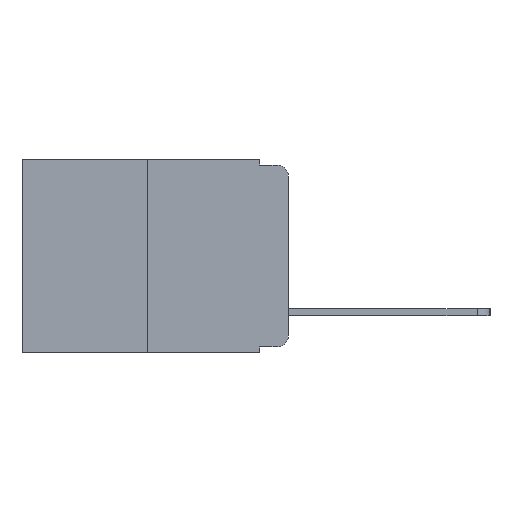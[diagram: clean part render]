
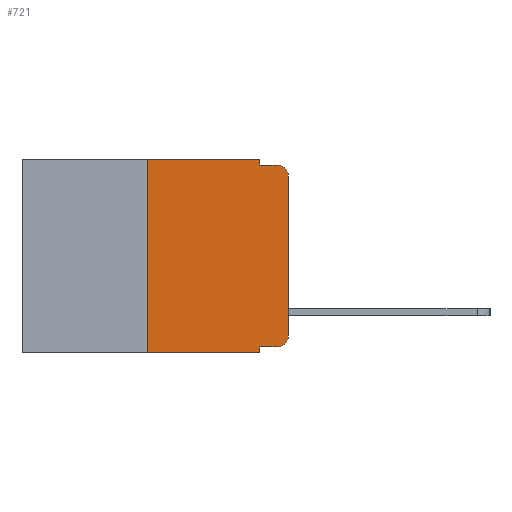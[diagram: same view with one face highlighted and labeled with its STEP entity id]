
A CAD part, left-side view. The second image highlights one B-rep face of the part: STEP entity #721.
In plain terms, the highlighted planar face has unit normal (-1, 0, 0).
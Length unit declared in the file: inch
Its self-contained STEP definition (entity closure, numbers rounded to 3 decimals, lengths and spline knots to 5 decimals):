
#57 = VECTOR ( 'NONE', #714, 39.37008 ) ;
#226 = ORIENTED_EDGE ( 'NONE', *, *, #11618, .F. ) ;
#510 = EDGE_LOOP ( 'NONE', ( #10164, #2613, #226, #4495, #8306, #1310, #3295, #8841, #8239, #8505 ) ) ;
#589 = DIRECTION ( 'NONE',  ( 0., -1., 0. ) ) ;
#631 = LINE ( 'NONE', #4341, #57 ) ;
#714 = DIRECTION ( 'NONE',  ( 0., -1., 0. ) ) ;
#721 = ADVANCED_FACE ( 'NONE', ( #5301 ), #7926, .F. ) ;
#779 = DIRECTION ( 'NONE',  ( -1., 0., 0. ) ) ;
#828 = VERTEX_POINT ( 'NONE', #9940 ) ;
#1003 = CARTESIAN_POINT ( 'NONE',  ( 0., 0.051, 0. ) ) ;
#1048 = DIRECTION ( 'NONE',  ( 0., 0., -1. ) ) ;
#1261 = CARTESIAN_POINT ( 'NONE',  ( 0., 0.25, 0. ) ) ;
#1300 = CARTESIAN_POINT ( 'NONE',  ( 0., 0.25, -0.343 ) ) ;
#1304 = VECTOR ( 'NONE', #7626, 39.37008 ) ;
#1310 = ORIENTED_EDGE ( 'NONE', *, *, #9658, .F. ) ;
#1512 = CIRCLE ( 'NONE', #4912, 0.02 ) ;
#1531 = EDGE_CURVE ( 'NONE', #2141, #9961, #1602, .T. ) ;
#1536 = EDGE_CURVE ( 'NONE', #2836, #5582, #8528, .T. ) ;
#1602 = LINE ( 'NONE', #2567, #10928 ) ;
#1744 = EDGE_CURVE ( 'NONE', #9961, #8989, #8674, .T. ) ;
#2134 = CARTESIAN_POINT ( 'NONE',  ( 0., 0., 0. ) ) ;
#2141 = VERTEX_POINT ( 'NONE', #7031 ) ;
#2186 = DIRECTION ( 'NONE',  ( 0., 0., 1. ) ) ;
#2297 = CARTESIAN_POINT ( 'NONE',  ( 0., 0.473, 0. ) ) ;
#2567 = CARTESIAN_POINT ( 'NONE',  ( 0., 0.051, -0.333 ) ) ;
#2613 = ORIENTED_EDGE ( 'NONE', *, *, #4461, .T. ) ;
#2667 = AXIS2_PLACEMENT_3D ( 'NONE', #9370, #7852, #7808 ) ;
#2836 = VERTEX_POINT ( 'NONE', #5036 ) ;
#3295 = ORIENTED_EDGE ( 'NONE', *, *, #5918, .T. ) ;
#3465 = DIRECTION ( 'NONE',  ( 0., -1., 0. ) ) ;
#3504 = CARTESIAN_POINT ( 'NONE',  ( 0., 0.02, -0.333 ) ) ;
#3606 = VECTOR ( 'NONE', #1048, 39.37008 ) ;
#3699 = EDGE_CURVE ( 'NONE', #2141, #8704, #11274, .T. ) ;
#3717 = VECTOR ( 'NONE', #589, 39.37008 ) ;
#3833 = VERTEX_POINT ( 'NONE', #7851 ) ;
#4313 = LINE ( 'NONE', #9675, #3717 ) ;
#4341 = CARTESIAN_POINT ( 'NONE',  ( 0., 0.051, -0.01 ) ) ;
#4461 = EDGE_CURVE ( 'NONE', #3833, #5516, #1512, .T. ) ;
#4495 = ORIENTED_EDGE ( 'NONE', *, *, #10710, .F. ) ;
#4684 = CARTESIAN_POINT ( 'NONE',  ( 0., 0.051, 0. ) ) ;
#4770 = EDGE_CURVE ( 'NONE', #8989, #3833, #5603, .T. ) ;
#4771 = CARTESIAN_POINT ( 'NONE',  ( 0., 0.051, 0. ) ) ;
#4912 = AXIS2_PLACEMENT_3D ( 'NONE', #6200, #779, #7119 ) ;
#5036 = CARTESIAN_POINT ( 'NONE',  ( 0., 0.25, 0. ) ) ;
#5054 = VECTOR ( 'NONE', #11173, 39.37008 ) ;
#5301 = FACE_OUTER_BOUND ( 'NONE', #510, .T. ) ;
#5516 = VERTEX_POINT ( 'NONE', #10612 ) ;
#5582 = VERTEX_POINT ( 'NONE', #1003 ) ;
#5603 = LINE ( 'NONE', #2134, #5054 ) ;
#5918 = EDGE_CURVE ( 'NONE', #9672, #8704, #4313, .T. ) ;
#6146 = CARTESIAN_POINT ( 'NONE',  ( 0., 0.051, -0.343 ) ) ;
#6200 = CARTESIAN_POINT ( 'NONE',  ( 0., 0.02, -0.03 ) ) ;
#6383 = DIRECTION ( 'NONE',  ( 0., 0., -1. ) ) ;
#6468 = DIRECTION ( 'NONE',  ( -1., 0., 0. ) ) ;
#6653 = CARTESIAN_POINT ( 'NONE',  ( 0., 0.02, -0.313 ) ) ;
#7031 = CARTESIAN_POINT ( 'NONE',  ( 0., 0.051, -0.333 ) ) ;
#7119 = DIRECTION ( 'NONE',  ( 0., 0., -1. ) ) ;
#7473 = VECTOR ( 'NONE', #2186, 39.37008 ) ;
#7626 = DIRECTION ( 'NONE',  ( 0., -1., 0. ) ) ;
#7808 = DIRECTION ( 'NONE',  ( 0., 0., -1. ) ) ;
#7851 = CARTESIAN_POINT ( 'NONE',  ( 0., 0., -0.03 ) ) ;
#7852 = DIRECTION ( 'NONE',  ( 1., 0., 0. ) ) ;
#7926 = PLANE ( 'NONE',  #2667 ) ;
#8239 = ORIENTED_EDGE ( 'NONE', *, *, #1531, .T. ) ;
#8306 = ORIENTED_EDGE ( 'NONE', *, *, #1536, .F. ) ;
#8369 = CARTESIAN_POINT ( 'NONE',  ( 0., 0., -0.313 ) ) ;
#8375 = DIRECTION ( 'NONE',  ( 0., 0., -1. ) ) ;
#8440 = LINE ( 'NONE', #4684, #3606 ) ;
#8505 = ORIENTED_EDGE ( 'NONE', *, *, #1744, .T. ) ;
#8528 = LINE ( 'NONE', #2297, #1304 ) ;
#8674 = CIRCLE ( 'NONE', #11295, 0.02 ) ;
#8704 = VERTEX_POINT ( 'NONE', #6146 ) ;
#8841 = ORIENTED_EDGE ( 'NONE', *, *, #3699, .F. ) ;
#8989 = VERTEX_POINT ( 'NONE', #8369 ) ;
#9370 = CARTESIAN_POINT ( 'NONE',  ( 0., 0.473, 0. ) ) ;
#9658 = EDGE_CURVE ( 'NONE', #9672, #2836, #9907, .T. ) ;
#9672 = VERTEX_POINT ( 'NONE', #1300 ) ;
#9675 = CARTESIAN_POINT ( 'NONE',  ( 0., 0.473, -0.343 ) ) ;
#9907 = LINE ( 'NONE', #1261, #7473 ) ;
#9940 = CARTESIAN_POINT ( 'NONE',  ( 0., 0.051, -0.01 ) ) ;
#9961 = VERTEX_POINT ( 'NONE', #3504 ) ;
#10164 = ORIENTED_EDGE ( 'NONE', *, *, #4770, .T. ) ;
#10612 = CARTESIAN_POINT ( 'NONE',  ( 0., 0.02, -0.01 ) ) ;
#10710 = EDGE_CURVE ( 'NONE', #5582, #828, #8440, .T. ) ;
#10928 = VECTOR ( 'NONE', #3465, 39.37008 ) ;
#10999 = VECTOR ( 'NONE', #8375, 39.37008 ) ;
#11173 = DIRECTION ( 'NONE',  ( 0., 0., 1. ) ) ;
#11274 = LINE ( 'NONE', #4771, #10999 ) ;
#11295 = AXIS2_PLACEMENT_3D ( 'NONE', #6653, #6468, #6383 ) ;
#11618 = EDGE_CURVE ( 'NONE', #828, #5516, #631, .T. ) ;
